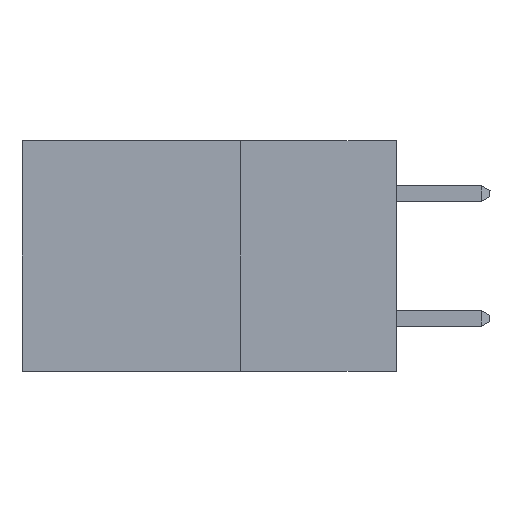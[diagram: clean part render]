
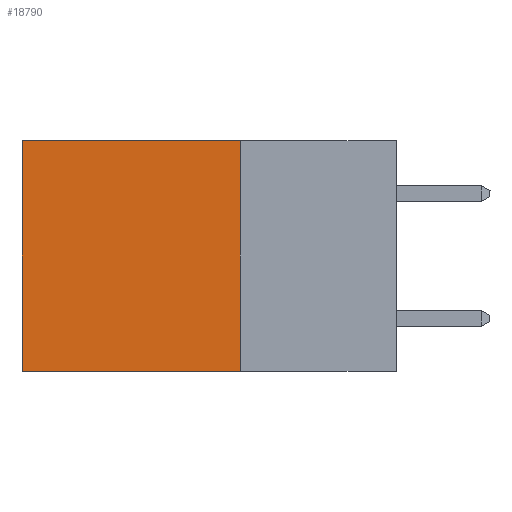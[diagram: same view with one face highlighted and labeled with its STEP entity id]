
A CAD part, left-side view. The second image highlights one B-rep face of the part: STEP entity #18790.
In plain terms, the highlighted planar face has unit normal (-1, 0, 0).
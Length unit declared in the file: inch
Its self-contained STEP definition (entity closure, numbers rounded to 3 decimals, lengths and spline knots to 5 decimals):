
#328 = VERTEX_POINT ( 'NONE', #2617 ) ;
#1531 = VECTOR ( 'NONE', #19142, 39.37008 ) ;
#1702 = LINE ( 'NONE', #21406, #15324 ) ;
#1835 = PLANE ( 'NONE',  #15524 ) ;
#2535 = CARTESIAN_POINT ( 'NONE',  ( 0.298, 0.25, 0. ) ) ;
#2617 = CARTESIAN_POINT ( 'NONE',  ( 0.298, 0.25, -0.37 ) ) ;
#3884 = EDGE_CURVE ( 'NONE', #19868, #16948, #1702, .T. ) ;
#3944 = DIRECTION ( 'NONE',  ( 0., 0., -1. ) ) ;
#4172 = ORIENTED_EDGE ( 'NONE', *, *, #20752, .F. ) ;
#5018 = CARTESIAN_POINT ( 'NONE',  ( 0.298, 0.25, 0. ) ) ;
#5367 = CARTESIAN_POINT ( 'NONE',  ( 0.298, 0.25, 0. ) ) ;
#6607 = ORIENTED_EDGE ( 'NONE', *, *, #3884, .T. ) ;
#7084 = ORIENTED_EDGE ( 'NONE', *, *, #7973, .F. ) ;
#7192 = DIRECTION ( 'NONE',  ( 0., 0., -1. ) ) ;
#7973 = EDGE_CURVE ( 'NONE', #328, #16948, #18967, .T. ) ;
#8186 = FACE_OUTER_BOUND ( 'NONE', #16947, .T. ) ;
#8638 = CARTESIAN_POINT ( 'NONE',  ( 0.298, 0.6, 0. ) ) ;
#9129 = CARTESIAN_POINT ( 'NONE',  ( 0.298, 0.25, 0. ) ) ;
#10812 = CARTESIAN_POINT ( 'NONE',  ( 0.298, 0.6, -0.37 ) ) ;
#11381 = VERTEX_POINT ( 'NONE', #2535 ) ;
#12902 = EDGE_CURVE ( 'NONE', #11381, #19868, #20264, .T. ) ;
#13024 = DIRECTION ( 'NONE',  ( 0., 1., 0. ) ) ;
#14387 = VECTOR ( 'NONE', #13024, 39.37008 ) ;
#15324 = VECTOR ( 'NONE', #3944, 39.37008 ) ;
#15524 = AXIS2_PLACEMENT_3D ( 'NONE', #5367, #17738, #7192 ) ;
#16516 = CARTESIAN_POINT ( 'NONE',  ( 0.298, 0.25, -0.37 ) ) ;
#16947 = EDGE_LOOP ( 'NONE', ( #6607, #7084, #4172, #21542 ) ) ;
#16948 = VERTEX_POINT ( 'NONE', #10812 ) ;
#17714 = LINE ( 'NONE', #9129, #18244 ) ;
#17738 = DIRECTION ( 'NONE',  ( 1., 0., 0. ) ) ;
#18244 = VECTOR ( 'NONE', #21361, 39.37008 ) ;
#18790 = ADVANCED_FACE ( 'NONE', ( #8186 ), #1835, .F. ) ;
#18967 = LINE ( 'NONE', #16516, #14387 ) ;
#19142 = DIRECTION ( 'NONE',  ( 0., 1., 0. ) ) ;
#19868 = VERTEX_POINT ( 'NONE', #8638 ) ;
#20264 = LINE ( 'NONE', #5018, #1531 ) ;
#20752 = EDGE_CURVE ( 'NONE', #11381, #328, #17714, .T. ) ;
#21361 = DIRECTION ( 'NONE',  ( 0., 0., -1. ) ) ;
#21406 = CARTESIAN_POINT ( 'NONE',  ( 0.298, 0.6, 0. ) ) ;
#21542 = ORIENTED_EDGE ( 'NONE', *, *, #12902, .T. ) ;
